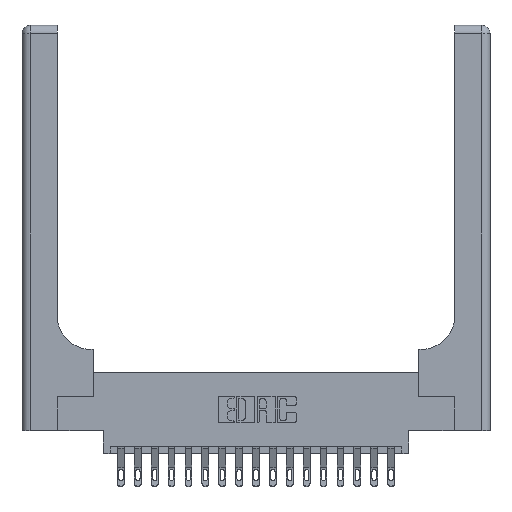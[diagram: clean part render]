
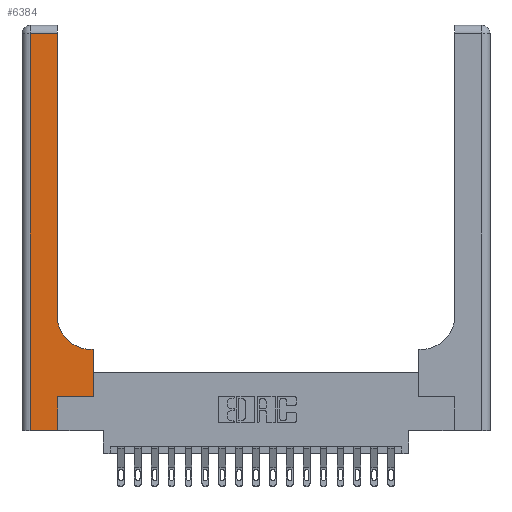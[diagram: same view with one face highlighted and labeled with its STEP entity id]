
A CAD part, top view. The second image highlights one B-rep face of the part: STEP entity #6384.
In plain terms, the highlighted planar face has unit normal (0, 0, 1).
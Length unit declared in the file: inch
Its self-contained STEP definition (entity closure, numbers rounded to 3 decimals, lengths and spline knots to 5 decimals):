
#97 = CARTESIAN_POINT ( 'NONE',  ( 0.51, 0.85, 0.37 ) ) ;
#378 = CARTESIAN_POINT ( 'NONE',  ( 0.265, 0.25, 0.37 ) ) ;
#703 = DIRECTION ( 'NONE',  ( -1., 0., 0. ) ) ;
#1087 = CARTESIAN_POINT ( 'NONE',  ( 0., 3., 0.37 ) ) ;
#1286 = CARTESIAN_POINT ( 'NONE',  ( 0.265, 0., 0.37 ) ) ;
#1357 = EDGE_CURVE ( 'NONE', #19136, #14311, #16928, .T. ) ;
#1662 = DIRECTION ( 'NONE',  ( 1., 0., 0. ) ) ;
#1856 = VECTOR ( 'NONE', #4771, 39.37008 ) ;
#2026 = CARTESIAN_POINT ( 'NONE',  ( 0.265, 0., 0.37 ) ) ;
#2443 = LINE ( 'NONE', #12629, #10251 ) ;
#2567 = LINE ( 'NONE', #10610, #18627 ) ;
#2645 = DIRECTION ( 'NONE',  ( 0., 0., -1. ) ) ;
#3394 = VERTEX_POINT ( 'NONE', #15597 ) ;
#3632 = DIRECTION ( 'NONE',  ( 0., 1., 0. ) ) ;
#4517 = VECTOR ( 'NONE', #20102, 39.37008 ) ;
#4713 = EDGE_CURVE ( 'NONE', #17158, #12791, #2443, .T. ) ;
#4771 = DIRECTION ( 'NONE',  ( 1., 0., 0. ) ) ;
#4822 = VERTEX_POINT ( 'NONE', #18990 ) ;
#4934 = CARTESIAN_POINT ( 'NONE',  ( 0.528, 0.25, 0.37 ) ) ;
#4985 = ORIENTED_EDGE ( 'NONE', *, *, #7994, .T. ) ;
#5066 = LINE ( 'NONE', #11590, #12378 ) ;
#5201 = EDGE_LOOP ( 'NONE', ( #17253, #16633, #16738, #7808, #4985, #9705, #14286, #5552, #7104 ) ) ;
#5552 = ORIENTED_EDGE ( 'NONE', *, *, #4713, .T. ) ;
#6056 = CARTESIAN_POINT ( 'NONE',  ( 0.265, 0.25, 0.37 ) ) ;
#6384 = ADVANCED_FACE ( 'NONE', ( #12368 ), #10413, .F. ) ;
#6734 = CARTESIAN_POINT ( 'NONE',  ( 0.51, 0.6, 0.37 ) ) ;
#7104 = ORIENTED_EDGE ( 'NONE', *, *, #19549, .T. ) ;
#7808 = ORIENTED_EDGE ( 'NONE', *, *, #12662, .T. ) ;
#7994 = EDGE_CURVE ( 'NONE', #20041, #19136, #14986, .T. ) ;
#8181 = CARTESIAN_POINT ( 'NONE',  ( 0.528, 0.6, 0.37 ) ) ;
#8685 = VECTOR ( 'NONE', #19014, 39.37008 ) ;
#9579 = LINE ( 'NONE', #11388, #17352 ) ;
#9705 = ORIENTED_EDGE ( 'NONE', *, *, #1357, .T. ) ;
#10251 = VECTOR ( 'NONE', #18856, 39.37008 ) ;
#10358 = VECTOR ( 'NONE', #3632, 39.37008 ) ;
#10413 = PLANE ( 'NONE',  #15882 ) ;
#10428 = EDGE_CURVE ( 'NONE', #14311, #17158, #9579, .T. ) ;
#10610 = CARTESIAN_POINT ( 'NONE',  ( 0.06, 3., 0.37 ) ) ;
#10876 = CARTESIAN_POINT ( 'NONE',  ( 0.06, 0., 0.37 ) ) ;
#10928 = VERTEX_POINT ( 'NONE', #12384 ) ;
#10976 = DIRECTION ( 'NONE',  ( 0., 0., -1. ) ) ;
#11347 = CIRCLE ( 'NONE', #13553, 0.25 ) ;
#11388 = CARTESIAN_POINT ( 'NONE',  ( 0.528, 0.25, 0.37 ) ) ;
#11590 = CARTESIAN_POINT ( 'NONE',  ( 0., 2.94, 0.37 ) ) ;
#12368 = FACE_OUTER_BOUND ( 'NONE', #5201, .T. ) ;
#12378 = VECTOR ( 'NONE', #703, 39.37008 ) ;
#12384 = CARTESIAN_POINT ( 'NONE',  ( 0.06, 2.94, 0.37 ) ) ;
#12629 = CARTESIAN_POINT ( 'NONE',  ( 0.26, 0.6, 0.37 ) ) ;
#12662 = EDGE_CURVE ( 'NONE', #17715, #20041, #14277, .T. ) ;
#12743 = EDGE_CURVE ( 'NONE', #3394, #4822, #12809, .T. ) ;
#12791 = VERTEX_POINT ( 'NONE', #6734 ) ;
#12809 = LINE ( 'NONE', #17487, #8685 ) ;
#13537 = DIRECTION ( 'NONE',  ( -1., 0., 0. ) ) ;
#13553 = AXIS2_PLACEMENT_3D ( 'NONE', #97, #10976, #1662 ) ;
#14277 = LINE ( 'NONE', #15648, #1856 ) ;
#14286 = ORIENTED_EDGE ( 'NONE', *, *, #10428, .T. ) ;
#14311 = VERTEX_POINT ( 'NONE', #4934 ) ;
#14986 = LINE ( 'NONE', #2026, #10358 ) ;
#15597 = CARTESIAN_POINT ( 'NONE',  ( 0.26, 0.85, 0.37 ) ) ;
#15648 = CARTESIAN_POINT ( 'NONE',  ( 0., 0., 0.37 ) ) ;
#15882 = AXIS2_PLACEMENT_3D ( 'NONE', #1087, #2645, #13537 ) ;
#16633 = ORIENTED_EDGE ( 'NONE', *, *, #18481, .T. ) ;
#16738 = ORIENTED_EDGE ( 'NONE', *, *, #20037, .T. ) ;
#16928 = LINE ( 'NONE', #6056, #4517 ) ;
#17158 = VERTEX_POINT ( 'NONE', #8181 ) ;
#17253 = ORIENTED_EDGE ( 'NONE', *, *, #12743, .T. ) ;
#17352 = VECTOR ( 'NONE', #19130, 39.37008 ) ;
#17487 = CARTESIAN_POINT ( 'NONE',  ( 0.26, 3., 0.37 ) ) ;
#17715 = VERTEX_POINT ( 'NONE', #10876 ) ;
#18481 = EDGE_CURVE ( 'NONE', #4822, #10928, #5066, .T. ) ;
#18627 = VECTOR ( 'NONE', #19889, 39.37008 ) ;
#18856 = DIRECTION ( 'NONE',  ( -1., 0., 0. ) ) ;
#18990 = CARTESIAN_POINT ( 'NONE',  ( 0.26, 2.94, 0.37 ) ) ;
#19014 = DIRECTION ( 'NONE',  ( 0., 1., 0. ) ) ;
#19130 = DIRECTION ( 'NONE',  ( 0., 1., 0. ) ) ;
#19136 = VERTEX_POINT ( 'NONE', #378 ) ;
#19549 = EDGE_CURVE ( 'NONE', #12791, #3394, #11347, .T. ) ;
#19889 = DIRECTION ( 'NONE',  ( 0., -1., 0. ) ) ;
#20037 = EDGE_CURVE ( 'NONE', #10928, #17715, #2567, .T. ) ;
#20041 = VERTEX_POINT ( 'NONE', #1286 ) ;
#20102 = DIRECTION ( 'NONE',  ( 1., 0., 0. ) ) ;
